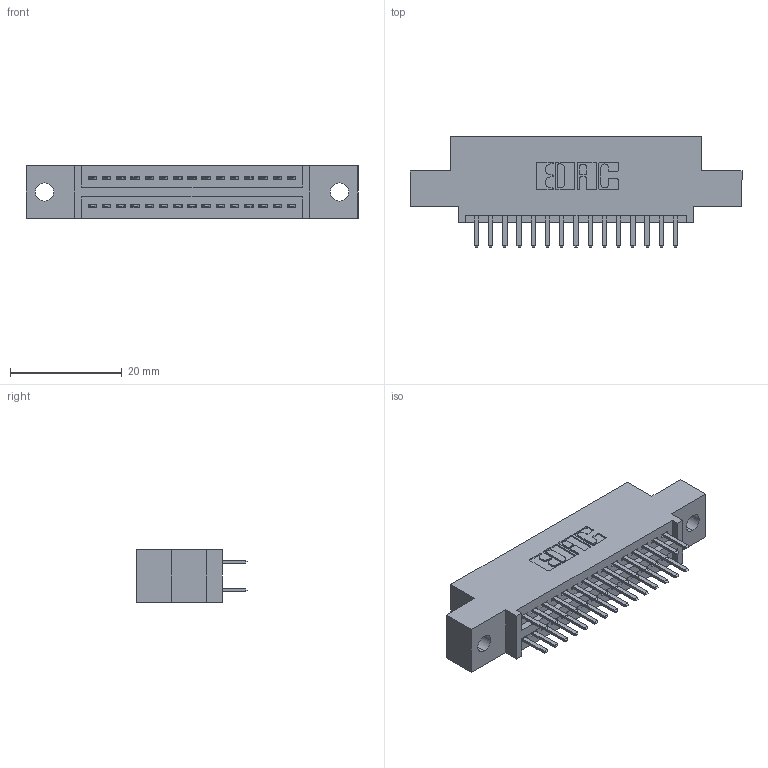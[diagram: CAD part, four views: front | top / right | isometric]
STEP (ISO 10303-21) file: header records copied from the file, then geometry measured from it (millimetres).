
FILE_DESCRIPTION (( 'STEP AP203' ), '1' );
FILE_NAME ('395-030-520-502.STEP', '2019-10-17T13:47:33', ( '' ), ( '' ), 'SwSTEP 2.0', 'SolidWorks 2016', '' );
FILE_SCHEMA (( 'CONFIG_CONTROL_DESIGN' ));
Length unit declared in the file: inch
Products named in the file (3): 395-030-520-502; 345 Part_0.110 Offset - 0.128 Dia; 345-292-001_345-293-120
Assembly tree (31 placements, depth 2):
  395-030-520-502
    345 Part_0.110 Offset - 0.128 Dia
    345-292-001_345-293-120  x30
Bounding box: 59.31 x 19.68 x 9.4 mm (x, y, z)
Volume: 5387.5 mm3; surface area: 7232.7 mm2
Topology: 31 solids, 31 shells, 1750 faces, 5063 edges, 3294 vertices
Faces by surface type: plane 1134, cylinder 616
Entity records: 15653 total; most frequent: CARTESIAN_POINT 2664, ORIENTED_EDGE 2586, DIRECTION 2369, EDGE_CURVE 1293, LINE 1097, VECTOR 1097, VERTEX_POINT 858, AXIS2_PLACEMENT_3D 636
